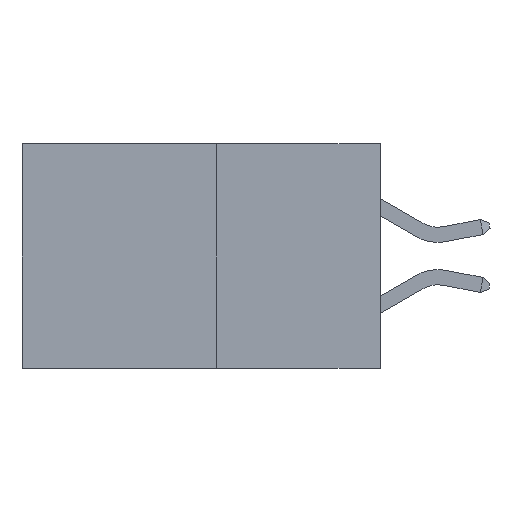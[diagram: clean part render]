
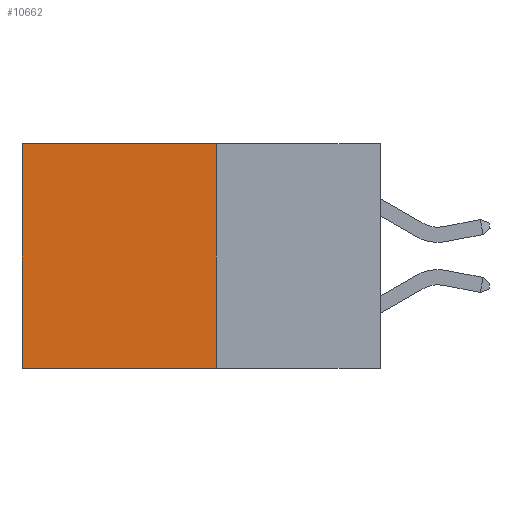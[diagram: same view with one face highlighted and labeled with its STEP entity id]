
A CAD part, left-side view. The second image highlights one B-rep face of the part: STEP entity #10662.
In plain terms, the highlighted planar face has unit normal (-1, 0, 0).
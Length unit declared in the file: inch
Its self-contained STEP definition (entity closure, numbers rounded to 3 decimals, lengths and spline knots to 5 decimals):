
#216 = ORIENTED_EDGE ( 'NONE', *, *, #1557, .T. ) ;
#945 = EDGE_LOOP ( 'NONE', ( #216, #2719, #7034, #24763 ) ) ;
#1557 = EDGE_CURVE ( 'NONE', #4378, #24864, #27270, .T. ) ;
#2719 = ORIENTED_EDGE ( 'NONE', *, *, #6596, .F. ) ;
#3982 = VECTOR ( 'NONE', #16775, 39.37008 ) ;
#4378 = VERTEX_POINT ( 'NONE', #21195 ) ;
#4679 = LINE ( 'NONE', #9865, #3982 ) ;
#5470 = CARTESIAN_POINT ( 'NONE',  ( 0.277, 0.59, -0.37 ) ) ;
#5499 = DIRECTION ( 'NONE',  ( 0., 0., -1. ) ) ;
#5572 = DIRECTION ( 'NONE',  ( 1., 0., 0. ) ) ;
#5677 = CARTESIAN_POINT ( 'NONE',  ( 0.277, 0.27, -0.37 ) ) ;
#6088 = PLANE ( 'NONE',  #12065 ) ;
#6164 = CARTESIAN_POINT ( 'NONE',  ( 0.277, 0.59, -0.37 ) ) ;
#6596 = EDGE_CURVE ( 'NONE', #17614, #24864, #7381, .T. ) ;
#7034 = ORIENTED_EDGE ( 'NONE', *, *, #18485, .F. ) ;
#7381 = LINE ( 'NONE', #14700, #17948 ) ;
#7571 = LINE ( 'NONE', #17792, #18840 ) ;
#9733 = FACE_OUTER_BOUND ( 'NONE', #945, .T. ) ;
#9865 = CARTESIAN_POINT ( 'NONE',  ( 0.277, 0.27, 0. ) ) ;
#10522 = CARTESIAN_POINT ( 'NONE',  ( 0.277, 0.27, 0. ) ) ;
#10662 = ADVANCED_FACE ( 'NONE', ( #9733 ), #6088, .F. ) ;
#12065 = AXIS2_PLACEMENT_3D ( 'NONE', #5677, #5572, #5499 ) ;
#14700 = CARTESIAN_POINT ( 'NONE',  ( 0.277, 0.27, -0.37 ) ) ;
#14948 = DIRECTION ( 'NONE',  ( 0., 1., 0. ) ) ;
#16775 = DIRECTION ( 'NONE',  ( 0., 1., 0. ) ) ;
#17614 = VERTEX_POINT ( 'NONE', #28621 ) ;
#17792 = CARTESIAN_POINT ( 'NONE',  ( 0.277, 0.27, -0.37 ) ) ;
#17948 = VECTOR ( 'NONE', #14948, 39.37008 ) ;
#18485 = EDGE_CURVE ( 'NONE', #26310, #17614, #7571, .T. ) ;
#18840 = VECTOR ( 'NONE', #20004, 39.37008 ) ;
#20004 = DIRECTION ( 'NONE',  ( 0., 0., -1. ) ) ;
#21195 = CARTESIAN_POINT ( 'NONE',  ( 0.277, 0.59, 0. ) ) ;
#21674 = VECTOR ( 'NONE', #27465, 39.37008 ) ;
#24763 = ORIENTED_EDGE ( 'NONE', *, *, #28670, .T. ) ;
#24864 = VERTEX_POINT ( 'NONE', #5470 ) ;
#26310 = VERTEX_POINT ( 'NONE', #10522 ) ;
#27270 = LINE ( 'NONE', #6164, #21674 ) ;
#27465 = DIRECTION ( 'NONE',  ( 0., 0., -1. ) ) ;
#28621 = CARTESIAN_POINT ( 'NONE',  ( 0.277, 0.27, -0.37 ) ) ;
#28670 = EDGE_CURVE ( 'NONE', #26310, #4378, #4679, .T. ) ;
